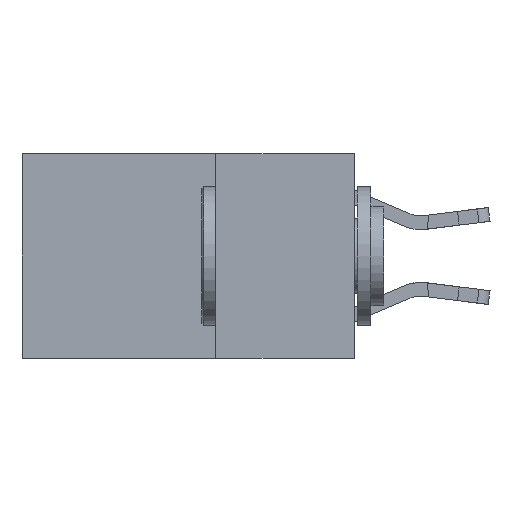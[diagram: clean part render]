
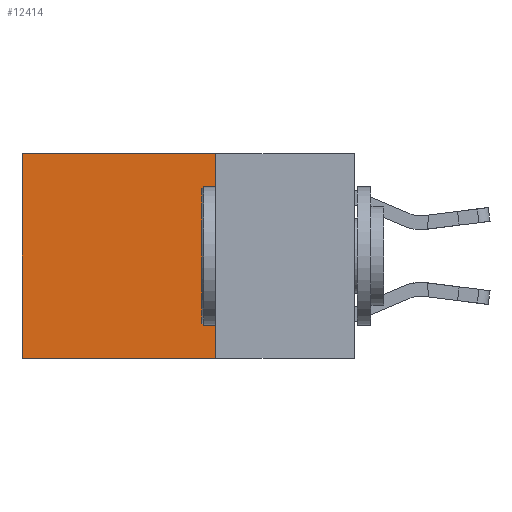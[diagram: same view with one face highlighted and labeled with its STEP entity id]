
A CAD part, left-side view. The second image highlights one B-rep face of the part: STEP entity #12414.
In plain terms, the highlighted planar face has unit normal (-1, 0, 0).
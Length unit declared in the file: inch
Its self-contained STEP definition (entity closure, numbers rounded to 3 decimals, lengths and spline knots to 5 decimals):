
#113 = CARTESIAN_POINT ( 'NONE',  ( 0.2625, 0.25, 0. ) ) ;
#879 = CARTESIAN_POINT ( 'NONE',  ( 0.2625, 0.6, 0. ) ) ;
#2316 = EDGE_CURVE ( 'NONE', #22217, #19999, #14627, .T. ) ;
#3407 = EDGE_CURVE ( 'NONE', #19999, #6698, #20418, .T. ) ;
#3589 = CARTESIAN_POINT ( 'NONE',  ( 0.2625, 0.25, 0. ) ) ;
#5092 = LINE ( 'NONE', #8738, #7067 ) ;
#5366 = LINE ( 'NONE', #3589, #22953 ) ;
#6698 = VERTEX_POINT ( 'NONE', #20145 ) ;
#7067 = VECTOR ( 'NONE', #15863, 39.37008 ) ;
#8254 = DIRECTION ( 'NONE',  ( 0., 0., -1. ) ) ;
#8738 = CARTESIAN_POINT ( 'NONE',  ( 0.2625, 0.25, -0.37 ) ) ;
#9348 = CARTESIAN_POINT ( 'NONE',  ( 0.2625, 0.25, -0.37 ) ) ;
#9524 = FACE_OUTER_BOUND ( 'NONE', #9918, .T. ) ;
#9636 = DIRECTION ( 'NONE',  ( 1., 0., 0. ) ) ;
#9902 = EDGE_CURVE ( 'NONE', #22217, #10047, #5366, .T. ) ;
#9918 = EDGE_LOOP ( 'NONE', ( #11629, #18331, #17387, #20116 ) ) ;
#10047 = VERTEX_POINT ( 'NONE', #9348 ) ;
#10275 = AXIS2_PLACEMENT_3D ( 'NONE', #11501, #9636, #16885 ) ;
#11501 = CARTESIAN_POINT ( 'NONE',  ( 0.2625, 0.25, 0. ) ) ;
#11629 = ORIENTED_EDGE ( 'NONE', *, *, #3407, .T. ) ;
#12414 = ADVANCED_FACE ( 'NONE', ( #9524 ), #15244, .F. ) ;
#13124 = CARTESIAN_POINT ( 'NONE',  ( 0.2625, 0.6, 0. ) ) ;
#14627 = LINE ( 'NONE', #14974, #15691 ) ;
#14974 = CARTESIAN_POINT ( 'NONE',  ( 0.2625, 0.25, 0. ) ) ;
#15244 = PLANE ( 'NONE',  #10275 ) ;
#15691 = VECTOR ( 'NONE', #18595, 39.37008 ) ;
#15863 = DIRECTION ( 'NONE',  ( 0., 1., 0. ) ) ;
#16885 = DIRECTION ( 'NONE',  ( 0., 0., -1. ) ) ;
#17387 = ORIENTED_EDGE ( 'NONE', *, *, #9902, .F. ) ;
#17440 = EDGE_CURVE ( 'NONE', #10047, #6698, #5092, .T. ) ;
#17870 = DIRECTION ( 'NONE',  ( 0., 0., -1. ) ) ;
#18331 = ORIENTED_EDGE ( 'NONE', *, *, #17440, .F. ) ;
#18595 = DIRECTION ( 'NONE',  ( 0., 1., 0. ) ) ;
#19999 = VERTEX_POINT ( 'NONE', #13124 ) ;
#20116 = ORIENTED_EDGE ( 'NONE', *, *, #2316, .T. ) ;
#20145 = CARTESIAN_POINT ( 'NONE',  ( 0.2625, 0.6, -0.37 ) ) ;
#20418 = LINE ( 'NONE', #879, #22111 ) ;
#22111 = VECTOR ( 'NONE', #8254, 39.37008 ) ;
#22217 = VERTEX_POINT ( 'NONE', #113 ) ;
#22953 = VECTOR ( 'NONE', #17870, 39.37008 ) ;
